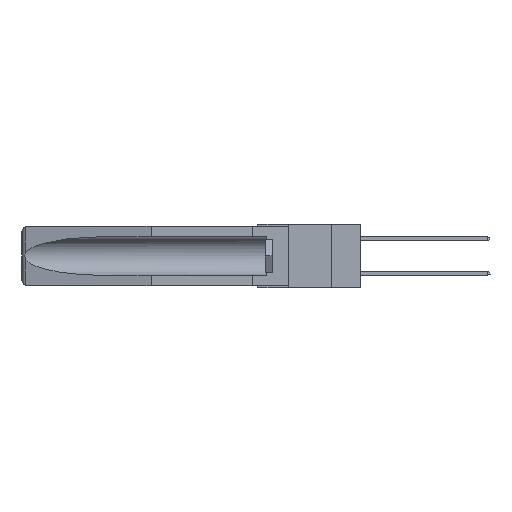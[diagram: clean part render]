
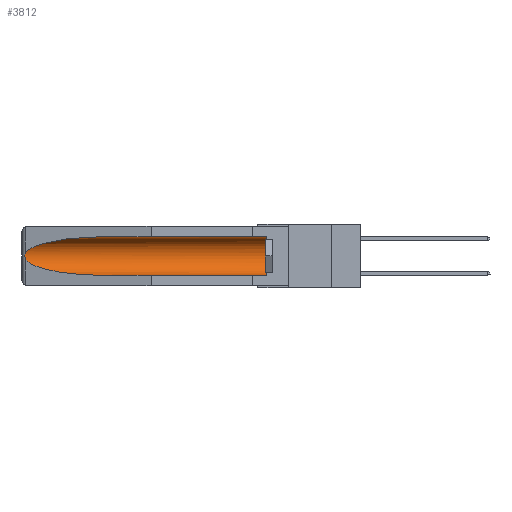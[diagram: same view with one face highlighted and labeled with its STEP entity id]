
A CAD part, left-side view. The second image highlights one B-rep face of the part: STEP entity #3812.
In plain terms, the highlighted cylindrical face has radius 2.857 mm (diameter 5.715 mm), a partial arc.
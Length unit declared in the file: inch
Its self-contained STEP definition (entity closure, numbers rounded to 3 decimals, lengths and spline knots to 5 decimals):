
#27 = ORIENTED_EDGE ( 'NONE', *, *, #4204, .T. ) ;
#648 = CARTESIAN_POINT ( 'NONE',  ( 0.2673, 1.53269, -0.17917 ) ) ;
#1182 = CARTESIAN_POINT ( 'NONE',  ( 0.155, 0.126, -0.059 ) ) ;
#1307 = CARTESIAN_POINT ( 'NONE',  ( 0.26537, 1.52718, -0.19328 ) ) ;
#2520 = VECTOR ( 'NONE', #26495, 39.37008 ) ;
#2781 = CARTESIAN_POINT ( 'NONE',  ( 0.26537, 1.52718, -0.19328 ) ) ;
#3812 = ADVANCED_FACE ( 'NONE', ( #28362 ), #20592, .F. ) ;
#4014 = VERTEX_POINT ( 'NONE', #30634 ) ;
#4204 = EDGE_CURVE ( 'NONE', #10439, #17334, #9963, .T. ) ;
#4744 = ORIENTED_EDGE ( 'NONE', *, *, #12086, .T. ) ;
#4773 = CARTESIAN_POINT ( 'NONE',  ( 0.25451, 1.48313, -0.24835 ) ) ;
#6979 = VERTEX_POINT ( 'NONE', #22293 ) ;
#7032 = CARTESIAN_POINT ( 'NONE',  ( 0.26597, 1.52961, -0.15275 ) ) ;
#7197 = EDGE_CURVE ( 'NONE', #17334, #6979, #16798, .T. ) ;
#7487 = ORIENTED_EDGE ( 'NONE', *, *, #29245, .T. ) ;
#8197 = CARTESIAN_POINT ( 'NONE',  ( 0.155, 1.07973, -0.059 ) ) ;
#9699 = CARTESIAN_POINT ( 'NONE',  ( 0.2673, 1.5327, -0.16383 ) ) ;
#9963 = B_SPLINE_CURVE_WITH_KNOTS ( 'NONE', 3,
 ( #21149, #7032, #23912, #9699, #28683, #14354, #648, #24010, #14561, #2781 ),
 .UNSPECIFIED., .F., .F.,
 ( 4, 2, 2, 2, 4 ),
 ( 0., 0.00029, 0.00058, 0.00087, 0.00117 ),
 .UNSPECIFIED. ) ;
#10439 = VERTEX_POINT ( 'NONE', #12285 ) ;
#10630 = DIRECTION ( 'NONE',  ( 0., 1., 0. ) ) ;
#12086 = EDGE_CURVE ( 'NONE', #25874, #4014, #27325, .T. ) ;
#12285 = CARTESIAN_POINT ( 'NONE',  ( 0.26537, 1.52718, -0.14972 ) ) ;
#12585 = CARTESIAN_POINT ( 'NONE',  ( 0.155, -0.30754, -0.059 ) ) ;
#13080 = EDGE_CURVE ( 'NONE', #4014, #10439, #25521, .T. ) ;
#14354 = CARTESIAN_POINT ( 'NONE',  ( 0.2675, 1.53308, -0.17534 ) ) ;
#14451 = CARTESIAN_POINT ( 'NONE',  ( 0.155, -0.30754, -0.284 ) ) ;
#14561 = CARTESIAN_POINT ( 'NONE',  ( 0.26597, 1.5296, -0.19026 ) ) ;
#14801 = CARTESIAN_POINT ( 'NONE',  ( 0.155, 1.07973, -0.284 ) ) ;
#15717 = DIRECTION ( 'NONE',  ( 0., 0., 1. ) ) ;
#16265 = CIRCLE ( 'NONE', #28086, 0.1125 ) ;
#16798 =( BOUNDED_CURVE ( )  B_SPLINE_CURVE ( 3, ( #18949, #4773, #24242, #14801 ),
 .UNSPECIFIED., .F., .F. ) 
 B_SPLINE_CURVE_WITH_KNOTS ( ( 4, 4 ),
 ( 0.1948, 1.5708 ),
 .UNSPECIFIED. ) 
 CURVE ( )  GEOMETRIC_REPRESENTATION_ITEM ( )  RATIONAL_B_SPLINE_CURVE ( ( 1., 0.848, 0.848, 1. ) ) 
 REPRESENTATION_ITEM ( '' )  );
#17245 = DIRECTION ( 'NONE',  ( 0., 1., 0. ) ) ;
#17334 = VERTEX_POINT ( 'NONE', #1307 ) ;
#17540 = CARTESIAN_POINT ( 'NONE',  ( 0.155, -0.30754, -0.1715 ) ) ;
#18118 = CARTESIAN_POINT ( 'NONE',  ( 0.25451, 1.48313, -0.09465 ) ) ;
#18949 = CARTESIAN_POINT ( 'NONE',  ( 0.26537, 1.52718, -0.19328 ) ) ;
#19920 = LINE ( 'NONE', #14451, #2520 ) ;
#20304 = VECTOR ( 'NONE', #10630, 39.37008 ) ;
#20339 = CARTESIAN_POINT ( 'NONE',  ( 0.21114, 1.30732, -0.059 ) ) ;
#20592 = CYLINDRICAL_SURFACE ( 'NONE', #28878, 0.1125 ) ;
#21149 = CARTESIAN_POINT ( 'NONE',  ( 0.26537, 1.52718, -0.14972 ) ) ;
#22293 = CARTESIAN_POINT ( 'NONE',  ( 0.155, 1.07973, -0.284 ) ) ;
#22418 = ORIENTED_EDGE ( 'NONE', *, *, #13080, .T. ) ;
#22886 = CARTESIAN_POINT ( 'NONE',  ( 0.155, 0.126, -0.284 ) ) ;
#23023 = CARTESIAN_POINT ( 'NONE',  ( 0.26537, 1.52718, -0.14972 ) ) ;
#23912 = CARTESIAN_POINT ( 'NONE',  ( 0.26654, 1.53092, -0.15636 ) ) ;
#24010 = CARTESIAN_POINT ( 'NONE',  ( 0.26655, 1.53094, -0.18657 ) ) ;
#24015 = VERTEX_POINT ( 'NONE', #22886 ) ;
#24242 = CARTESIAN_POINT ( 'NONE',  ( 0.21114, 1.30732, -0.284 ) ) ;
#25168 = CARTESIAN_POINT ( 'NONE',  ( 0.155, 0.126, -0.1715 ) ) ;
#25521 =( BOUNDED_CURVE ( )  B_SPLINE_CURVE ( 3, ( #8197, #20339, #18118, #23023 ),
 .UNSPECIFIED., .F., .F. ) 
 B_SPLINE_CURVE_WITH_KNOTS ( ( 4, 4 ),
 ( 4.71239, 6.08839 ),
 .UNSPECIFIED. ) 
 CURVE ( )  GEOMETRIC_REPRESENTATION_ITEM ( )  RATIONAL_B_SPLINE_CURVE ( ( 1., 0.848, 0.848, 1. ) ) 
 REPRESENTATION_ITEM ( '' )  );
#25697 = ORIENTED_EDGE ( 'NONE', *, *, #7197, .T. ) ;
#25874 = VERTEX_POINT ( 'NONE', #1182 ) ;
#26495 = DIRECTION ( 'NONE',  ( 0., 1., 0. ) ) ;
#26686 = DIRECTION ( 'NONE',  ( 0., 0., 1. ) ) ;
#27080 = EDGE_LOOP ( 'NONE', ( #22418, #27, #25697, #27350, #7487, #4744 ) ) ;
#27325 = LINE ( 'NONE', #12585, #20304 ) ;
#27350 = ORIENTED_EDGE ( 'NONE', *, *, #30515, .F. ) ;
#27560 = DIRECTION ( 'NONE',  ( 0., -1., 0. ) ) ;
#28086 = AXIS2_PLACEMENT_3D ( 'NONE', #25168, #27560, #15717 ) ;
#28362 = FACE_OUTER_BOUND ( 'NONE', #27080, .T. ) ;
#28683 = CARTESIAN_POINT ( 'NONE',  ( 0.2675, 1.53308, -0.16763 ) ) ;
#28878 = AXIS2_PLACEMENT_3D ( 'NONE', #17540, #17245, #26686 ) ;
#29245 = EDGE_CURVE ( 'NONE', #24015, #25874, #16265, .T. ) ;
#30515 = EDGE_CURVE ( 'NONE', #24015, #6979, #19920, .T. ) ;
#30634 = CARTESIAN_POINT ( 'NONE',  ( 0.155, 1.07973, -0.059 ) ) ;
